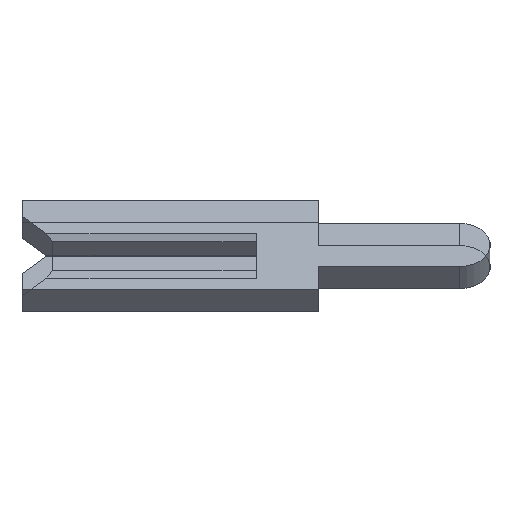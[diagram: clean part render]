
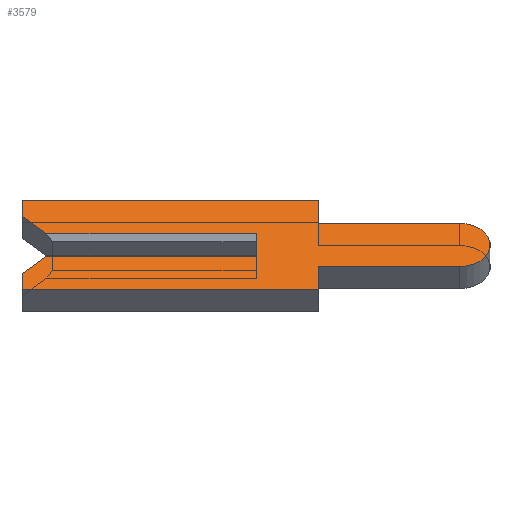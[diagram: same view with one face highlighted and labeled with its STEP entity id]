
A CAD part, left-side view. The second image highlights one B-rep face of the part: STEP entity #3579.
In plain terms, the highlighted face is planar.
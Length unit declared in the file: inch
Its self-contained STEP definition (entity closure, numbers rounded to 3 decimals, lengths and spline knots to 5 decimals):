
#5 = VECTOR ( 'NONE', #282, 39.37008 ) ;
#13 = VERTEX_POINT ( 'NONE', #2185 ) ;
#42 = VECTOR ( 'NONE', #3966, 39.37008 ) ;
#79 = VERTEX_POINT ( 'NONE', #3315 ) ;
#183 = CARTESIAN_POINT ( 'NONE',  ( -0.01, 0.134, 0.01 ) ) ;
#187 = VECTOR ( 'NONE', #2756, 39.37008 ) ;
#191 = LINE ( 'NONE', #3581, #5 ) ;
#219 = CARTESIAN_POINT ( 'NONE',  ( -0.01, 0., -0.01 ) ) ;
#282 = DIRECTION ( 'NONE',  ( 0., 0., -1. ) ) ;
#323 = EDGE_CURVE ( 'NONE', #1187, #1719, #1542, .T. ) ;
#327 = CARTESIAN_POINT ( 'NONE',  ( -0.01, 0.15, -0.026 ) ) ;
#328 = LINE ( 'NONE', #1976, #2849 ) ;
#405 = VERTEX_POINT ( 'NONE', #2883 ) ;
#455 = VERTEX_POINT ( 'NONE', #327 ) ;
#461 = CARTESIAN_POINT ( 'NONE',  ( -0.01, -0.1305, -0.0195 ) ) ;
#470 = ORIENTED_EDGE ( 'NONE', *, *, #3133, .F. ) ;
#631 = LINE ( 'NONE', #2087, #1410 ) ;
#747 = VECTOR ( 'NONE', #3844, 39.37008 ) ;
#756 = CARTESIAN_POINT ( 'NONE',  ( -0.01, -0.04, 0.0195 ) ) ;
#792 = DIRECTION ( 'NONE',  ( 0., 0., -1. ) ) ;
#911 = CARTESIAN_POINT ( 'NONE',  ( -0.01, 0.15, 0.04 ) ) ;
#953 = CARTESIAN_POINT ( 'NONE',  ( -0.01, 0.134, -0.01 ) ) ;
#977 = LINE ( 'NONE', #1017, #1833 ) ;
#983 = ORIENTED_EDGE ( 'NONE', *, *, #3378, .F. ) ;
#1017 = CARTESIAN_POINT ( 'NONE',  ( -0.01, -0.1305, -0.01 ) ) ;
#1115 = CARTESIAN_POINT ( 'NONE',  ( -0.01, -0.04, -0.04 ) ) ;
#1187 = VERTEX_POINT ( 'NONE', #2643 ) ;
#1204 = VECTOR ( 'NONE', #1318, 39.37008 ) ;
#1286 = VERTEX_POINT ( 'NONE', #2261 ) ;
#1315 = ORIENTED_EDGE ( 'NONE', *, *, #2048, .F. ) ;
#1318 = DIRECTION ( 'NONE',  ( 0., -1., 0. ) ) ;
#1338 = ORIENTED_EDGE ( 'NONE', *, *, #2797, .F. ) ;
#1384 = VERTEX_POINT ( 'NONE', #461 ) ;
#1396 = CARTESIAN_POINT ( 'NONE',  ( -0.01, 0.1305, 0.0065 ) ) ;
#1410 = VECTOR ( 'NONE', #2482, 39.37008 ) ;
#1435 = LINE ( 'NONE', #4180, #1204 ) ;
#1443 = LINE ( 'NONE', #2053, #187 ) ;
#1542 = LINE ( 'NONE', #756, #42 ) ;
#1660 = PLANE ( 'NONE',  #3669 ) ;
#1673 = DIRECTION ( 'NONE',  ( 0., 0., 1. ) ) ;
#1719 = VERTEX_POINT ( 'NONE', #1862 ) ;
#1750 = EDGE_CURVE ( 'NONE', #1719, #1384, #2497, .T. ) ;
#1833 = VECTOR ( 'NONE', #4024, 39.37008 ) ;
#1836 = DIRECTION ( 'NONE',  ( 0., 0., -1. ) ) ;
#1857 = DIRECTION ( 'NONE',  ( 0., 0., -1. ) ) ;
#1862 = CARTESIAN_POINT ( 'NONE',  ( -0.01, -0.1305, 0.0195 ) ) ;
#1876 = DIRECTION ( 'NONE',  ( 1., 0., 0. ) ) ;
#1976 = CARTESIAN_POINT ( 'NONE',  ( -0.01, 0.15, -0.026 ) ) ;
#1999 = DIRECTION ( 'NONE',  ( 0., -1., 0. ) ) ;
#2008 = VERTEX_POINT ( 'NONE', #911 ) ;
#2014 = ORIENTED_EDGE ( 'NONE', *, *, #4500, .F. ) ;
#2048 = EDGE_CURVE ( 'NONE', #79, #455, #328, .T. ) ;
#2053 = CARTESIAN_POINT ( 'NONE',  ( -0.01, 0.15, 0.026 ) ) ;
#2087 = CARTESIAN_POINT ( 'NONE',  ( -0.01, 0.15, -0.04 ) ) ;
#2149 = VERTEX_POINT ( 'NONE', #2694 ) ;
#2163 = VECTOR ( 'NONE', #4377, 39.37008 ) ;
#2171 = VECTOR ( 'NONE', #4503, 39.37008 ) ;
#2174 = EDGE_LOOP ( 'NONE', ( #2621, #2793, #3331, #983, #1315, #2976, #2014, #2463, #2366, #2579, #2743, #470, #1338, #3322 ) ) ;
#2185 = CARTESIAN_POINT ( 'NONE',  ( -0.01, -0.04, -0.0195 ) ) ;
#2202 = CARTESIAN_POINT ( 'NONE',  ( -0.01, 0., 0.01 ) ) ;
#2261 = CARTESIAN_POINT ( 'NONE',  ( -0.01, 0.15, 0.026 ) ) ;
#2345 = DIRECTION ( 'NONE',  ( 0., 0., 1. ) ) ;
#2366 = ORIENTED_EDGE ( 'NONE', *, *, #1750, .F. ) ;
#2405 = EDGE_CURVE ( 'NONE', #2504, #3898, #3210, .T. ) ;
#2463 = ORIENTED_EDGE ( 'NONE', *, *, #2561, .F. ) ;
#2482 = DIRECTION ( 'NONE',  ( 0., 1., 0. ) ) ;
#2497 = CIRCLE ( 'NONE', #4518, 0.0195 ) ;
#2504 = VERTEX_POINT ( 'NONE', #183 ) ;
#2561 = EDGE_CURVE ( 'NONE', #1384, #13, #3890, .T. ) ;
#2579 = ORIENTED_EDGE ( 'NONE', *, *, #323, .F. ) ;
#2621 = ORIENTED_EDGE ( 'NONE', *, *, #2405, .T. ) ;
#2643 = CARTESIAN_POINT ( 'NONE',  ( -0.01, -0.04, 0.0195 ) ) ;
#2694 = CARTESIAN_POINT ( 'NONE',  ( -0.01, -0.04, -0.04 ) ) ;
#2712 = EDGE_CURVE ( 'NONE', #3426, #3898, #3267, .T. ) ;
#2731 = CARTESIAN_POINT ( 'NONE',  ( -0.01, 0.15, 0.01 ) ) ;
#2743 = ORIENTED_EDGE ( 'NONE', *, *, #3778, .F. ) ;
#2756 = DIRECTION ( 'NONE',  ( 0., 0., 1. ) ) ;
#2793 = ORIENTED_EDGE ( 'NONE', *, *, #2712, .F. ) ;
#2797 = EDGE_CURVE ( 'NONE', #1286, #2008, #1443, .T. ) ;
#2849 = VECTOR ( 'NONE', #2345, 39.37008 ) ;
#2853 = VERTEX_POINT ( 'NONE', #953 ) ;
#2883 = CARTESIAN_POINT ( 'NONE',  ( -0.01, -0.04, 0.04 ) ) ;
#2917 = LINE ( 'NONE', #1396, #2163 ) ;
#2953 = DIRECTION ( 'NONE',  ( 1., 0., 0. ) ) ;
#2976 = ORIENTED_EDGE ( 'NONE', *, *, #4332, .F. ) ;
#3133 = EDGE_CURVE ( 'NONE', #2008, #405, #1435, .T. ) ;
#3159 = VECTOR ( 'NONE', #1673, 39.37008 ) ;
#3210 = LINE ( 'NONE', #2731, #4281 ) ;
#3267 = LINE ( 'NONE', #4244, #3159 ) ;
#3315 = CARTESIAN_POINT ( 'NONE',  ( -0.01, 0.15, -0.04 ) ) ;
#3322 = ORIENTED_EDGE ( 'NONE', *, *, #3873, .F. ) ;
#3331 = ORIENTED_EDGE ( 'NONE', *, *, #3700, .F. ) ;
#3378 = EDGE_CURVE ( 'NONE', #455, #2853, #3503, .T. ) ;
#3426 = VERTEX_POINT ( 'NONE', #219 ) ;
#3503 = LINE ( 'NONE', #3509, #747 ) ;
#3509 = CARTESIAN_POINT ( 'NONE',  ( -0.01, 0.1305, -0.0065 ) ) ;
#3579 = ADVANCED_FACE ( 'NONE', ( #4231 ), #1660, .F. ) ;
#3581 = CARTESIAN_POINT ( 'NONE',  ( -0.01, -0.04, 0.04 ) ) ;
#3669 = AXIS2_PLACEMENT_3D ( 'NONE', #4203, #2953, #1836 ) ;
#3693 = CARTESIAN_POINT ( 'NONE',  ( -0.01, -0.1305, 0. ) ) ;
#3700 = EDGE_CURVE ( 'NONE', #2853, #3426, #977, .T. ) ;
#3756 = VECTOR ( 'NONE', #1857, 39.37008 ) ;
#3764 = CARTESIAN_POINT ( 'NONE',  ( -0.01, -0.04, -0.0195 ) ) ;
#3778 = EDGE_CURVE ( 'NONE', #405, #1187, #191, .T. ) ;
#3844 = DIRECTION ( 'NONE',  ( 0., -0.707, 0.707 ) ) ;
#3873 = EDGE_CURVE ( 'NONE', #2504, #1286, #2917, .T. ) ;
#3890 = LINE ( 'NONE', #3764, #2171 ) ;
#3898 = VERTEX_POINT ( 'NONE', #2202 ) ;
#3966 = DIRECTION ( 'NONE',  ( 0., -1., 0. ) ) ;
#4024 = DIRECTION ( 'NONE',  ( 0., -1., 0. ) ) ;
#4180 = CARTESIAN_POINT ( 'NONE',  ( -0.01, 0.15, 0.04 ) ) ;
#4203 = CARTESIAN_POINT ( 'NONE',  ( -0.01, -0.1305, 0. ) ) ;
#4231 = FACE_OUTER_BOUND ( 'NONE', #2174, .T. ) ;
#4244 = CARTESIAN_POINT ( 'NONE',  ( -0.01, 0., 0.0065 ) ) ;
#4281 = VECTOR ( 'NONE', #1999, 39.37008 ) ;
#4332 = EDGE_CURVE ( 'NONE', #2149, #79, #631, .T. ) ;
#4363 = LINE ( 'NONE', #1115, #3756 ) ;
#4377 = DIRECTION ( 'NONE',  ( 0., 0.707, 0.707 ) ) ;
#4500 = EDGE_CURVE ( 'NONE', #13, #2149, #4363, .T. ) ;
#4503 = DIRECTION ( 'NONE',  ( 0., 1., 0. ) ) ;
#4518 = AXIS2_PLACEMENT_3D ( 'NONE', #3693, #1876, #792 ) ;
